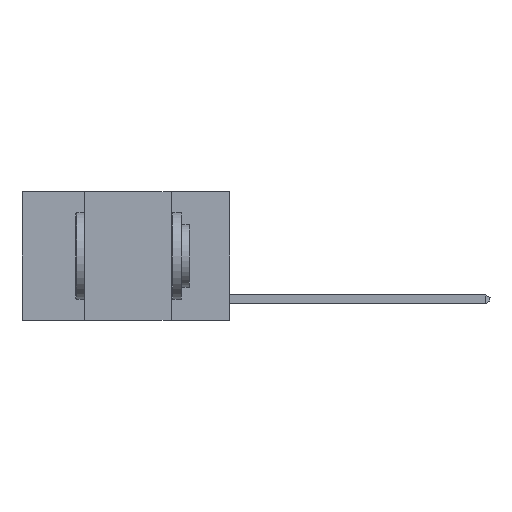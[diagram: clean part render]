
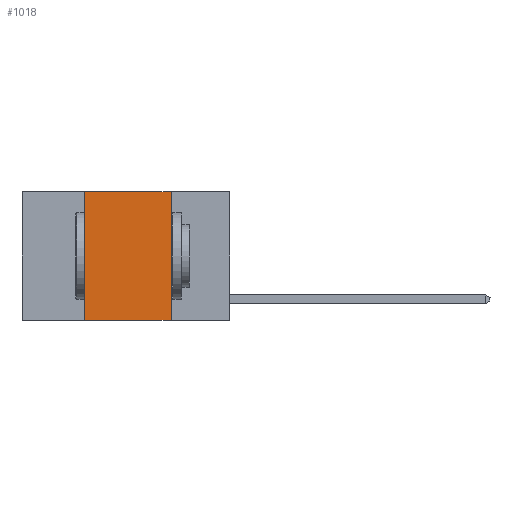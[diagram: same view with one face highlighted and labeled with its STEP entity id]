
A CAD part, left-side view. The second image highlights one B-rep face of the part: STEP entity #1018.
In plain terms, the highlighted planar face has unit normal (-1, 0, 0).
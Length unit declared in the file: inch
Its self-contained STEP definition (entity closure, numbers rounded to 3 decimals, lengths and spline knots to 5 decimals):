
#188 = CARTESIAN_POINT ( 'NONE',  ( 0., 0.42, 0. ) ) ;
#1018 = ADVANCED_FACE ( 'NONE', ( #3355 ), #7721, .F. ) ;
#1390 = VECTOR ( 'NONE', #7924, 39.37008 ) ;
#1508 = DIRECTION ( 'NONE',  ( 0., 0., 1. ) ) ;
#1543 = LINE ( 'NONE', #188, #12852 ) ;
#1674 = CARTESIAN_POINT ( 'NONE',  ( 0., 0.42, -0.37 ) ) ;
#2283 = CARTESIAN_POINT ( 'NONE',  ( 0., 0.17, 0. ) ) ;
#2464 = CARTESIAN_POINT ( 'NONE',  ( 0., 0.6, 0. ) ) ;
#3355 = FACE_OUTER_BOUND ( 'NONE', #3458, .T. ) ;
#3458 = EDGE_LOOP ( 'NONE', ( #7373, #7027, #6868, #6996 ) ) ;
#3851 = DIRECTION ( 'NONE',  ( 0., -1., 0. ) ) ;
#4675 = CARTESIAN_POINT ( 'NONE',  ( 0., 0.17, -0.37 ) ) ;
#5758 = VERTEX_POINT ( 'NONE', #1674 ) ;
#6061 = CARTESIAN_POINT ( 'NONE',  ( 0., 0.6, -0.37 ) ) ;
#6868 = ORIENTED_EDGE ( 'NONE', *, *, #9366, .F. ) ;
#6996 = ORIENTED_EDGE ( 'NONE', *, *, #10115, .T. ) ;
#7027 = ORIENTED_EDGE ( 'NONE', *, *, #14064, .F. ) ;
#7091 = EDGE_CURVE ( 'NONE', #7177, #8506, #12407, .T. ) ;
#7177 = VERTEX_POINT ( 'NONE', #8017 ) ;
#7373 = ORIENTED_EDGE ( 'NONE', *, *, #7091, .F. ) ;
#7626 = DIRECTION ( 'NONE',  ( 0., 0., -1. ) ) ;
#7643 = DIRECTION ( 'NONE',  ( 1., 0., 0. ) ) ;
#7721 = PLANE ( 'NONE',  #12994 ) ;
#7924 = DIRECTION ( 'NONE',  ( 0., 0., -1. ) ) ;
#8017 = CARTESIAN_POINT ( 'NONE',  ( 0., 0.17, 0. ) ) ;
#8337 = VECTOR ( 'NONE', #9236, 39.37008 ) ;
#8428 = VERTEX_POINT ( 'NONE', #12470 ) ;
#8506 = VERTEX_POINT ( 'NONE', #4675 ) ;
#8950 = CARTESIAN_POINT ( 'NONE',  ( 0., 0.6, 0. ) ) ;
#9236 = DIRECTION ( 'NONE',  ( 0., -1., 0. ) ) ;
#9335 = LINE ( 'NONE', #6061, #12343 ) ;
#9366 = EDGE_CURVE ( 'NONE', #5758, #8428, #1543, .T. ) ;
#10115 = EDGE_CURVE ( 'NONE', #5758, #8506, #9335, .T. ) ;
#11726 = LINE ( 'NONE', #2464, #8337 ) ;
#12343 = VECTOR ( 'NONE', #3851, 39.37008 ) ;
#12407 = LINE ( 'NONE', #2283, #1390 ) ;
#12470 = CARTESIAN_POINT ( 'NONE',  ( 0., 0.42, 0. ) ) ;
#12852 = VECTOR ( 'NONE', #1508, 39.37008 ) ;
#12994 = AXIS2_PLACEMENT_3D ( 'NONE', #8950, #7643, #7626 ) ;
#14064 = EDGE_CURVE ( 'NONE', #8428, #7177, #11726, .T. ) ;
